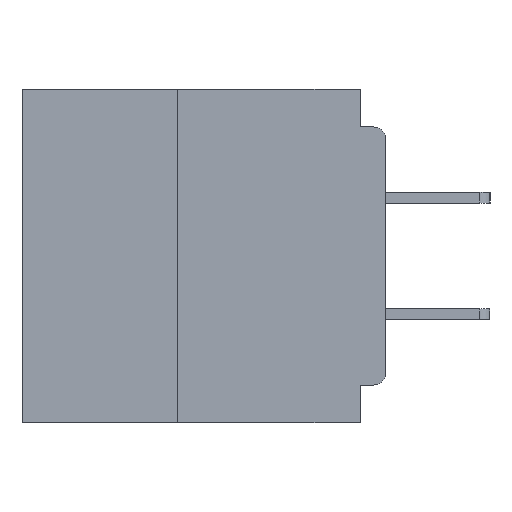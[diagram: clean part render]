
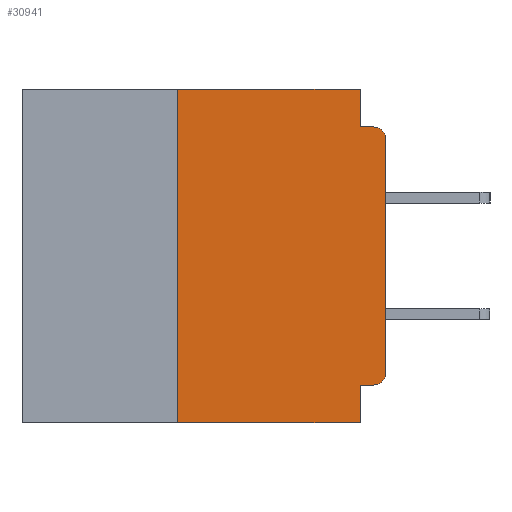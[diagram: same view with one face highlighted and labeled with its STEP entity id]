
A CAD part, left-side view. The second image highlights one B-rep face of the part: STEP entity #30941.
In plain terms, the highlighted planar face has unit normal (-1, 0, 0).
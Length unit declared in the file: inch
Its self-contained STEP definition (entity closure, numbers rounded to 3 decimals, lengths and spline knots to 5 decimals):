
#73 = EDGE_CURVE ( 'NONE', #10631, #47198, #45002, .T. ) ;
#103 = VERTEX_POINT ( 'NONE', #47614 ) ;
#166 = EDGE_CURVE ( 'NONE', #38303, #42740, #32128, .T. ) ;
#381 = ORIENTED_EDGE ( 'NONE', *, *, #36331, .F. ) ;
#466 = DIRECTION ( 'NONE',  ( 0., -1., 0. ) ) ;
#720 = EDGE_CURVE ( 'NONE', #40100, #45804, #36971, .T. ) ;
#778 = VECTOR ( 'NONE', #30493, 39.37008 ) ;
#966 = DIRECTION ( 'NONE',  ( 0., -1., 0. ) ) ;
#1097 = VERTEX_POINT ( 'NONE', #38771 ) ;
#1276 = LINE ( 'NONE', #42677, #31712 ) ;
#1330 = DIRECTION ( 'NONE',  ( -1., 0., 0. ) ) ;
#1372 = VERTEX_POINT ( 'NONE', #24798 ) ;
#2647 = DIRECTION ( 'NONE',  ( 0., 0., -1. ) ) ;
#2910 = ORIENTED_EDGE ( 'NONE', *, *, #73, .F. ) ;
#3764 = ORIENTED_EDGE ( 'NONE', *, *, #27282, .F. ) ;
#5622 = DIRECTION ( 'NONE',  ( 0., 0., 1. ) ) ;
#5649 = PLANE ( 'NONE',  #48093 ) ;
#5783 = CARTESIAN_POINT ( 'NONE',  ( 0., 0.25, -0.4 ) ) ;
#6669 = ORIENTED_EDGE ( 'NONE', *, *, #6833, .F. ) ;
#6833 = EDGE_CURVE ( 'NONE', #40100, #103, #1276, .T. ) ;
#9075 = VERTEX_POINT ( 'NONE', #46706 ) ;
#9662 = DIRECTION ( 'NONE',  ( 1., 0., 0. ) ) ;
#9680 = CARTESIAN_POINT ( 'NONE',  ( 0., 0., 0. ) ) ;
#10631 = VERTEX_POINT ( 'NONE', #31470 ) ;
#12347 = CARTESIAN_POINT ( 'NONE',  ( 0., 0.437, 0. ) ) ;
#13268 = CARTESIAN_POINT ( 'NONE',  ( 0., 0.437, -0.4 ) ) ;
#19511 = ORIENTED_EDGE ( 'NONE', *, *, #36813, .F. ) ;
#20322 = CARTESIAN_POINT ( 'NONE',  ( 0., 0.031, -0.4 ) ) ;
#23499 = LINE ( 'NONE', #5783, #43173 ) ;
#24798 = CARTESIAN_POINT ( 'NONE',  ( 0., 0.25, 0. ) ) ;
#24880 = ORIENTED_EDGE ( 'NONE', *, *, #720, .T. ) ;
#25169 = CARTESIAN_POINT ( 'NONE',  ( 0., 0.015, -0.06 ) ) ;
#25538 = DIRECTION ( 'NONE',  ( -1., 0., 0. ) ) ;
#26709 = VECTOR ( 'NONE', #37315, 39.37008 ) ;
#26934 = ORIENTED_EDGE ( 'NONE', *, *, #40611, .T. ) ;
#27282 = EDGE_CURVE ( 'NONE', #9075, #10631, #41637, .T. ) ;
#28320 = LINE ( 'NONE', #20322, #48008 ) ;
#28682 = AXIS2_PLACEMENT_3D ( 'NONE', #25169, #1330, #29096 ) ;
#28920 = EDGE_CURVE ( 'NONE', #45804, #1097, #38390, .T. ) ;
#29096 = DIRECTION ( 'NONE',  ( 0., 0., -1. ) ) ;
#29609 = VECTOR ( 'NONE', #466, 39.37008 ) ;
#29658 = CARTESIAN_POINT ( 'NONE',  ( 0., 0.015, -0.355 ) ) ;
#30235 = CARTESIAN_POINT ( 'NONE',  ( 0., 0.015, -0.045 ) ) ;
#30493 = DIRECTION ( 'NONE',  ( 0., 0., -1. ) ) ;
#30941 = ADVANCED_FACE ( 'NONE', ( #43107 ), #5649, .F. ) ;
#31470 = CARTESIAN_POINT ( 'NONE',  ( 0., 0.031, -0.045 ) ) ;
#31631 = EDGE_LOOP ( 'NONE', ( #38741, #26934, #2910, #3764, #381, #41489, #33627, #19511, #6669, #24880 ) ) ;
#31712 = VECTOR ( 'NONE', #38874, 39.37008 ) ;
#32128 = LINE ( 'NONE', #13268, #40053 ) ;
#33411 = CARTESIAN_POINT ( 'NONE',  ( 0., 0.437, 0. ) ) ;
#33627 = ORIENTED_EDGE ( 'NONE', *, *, #166, .T. ) ;
#34549 = VECTOR ( 'NONE', #47604, 39.37008 ) ;
#36331 = EDGE_CURVE ( 'NONE', #1372, #9075, #40046, .T. ) ;
#36813 = EDGE_CURVE ( 'NONE', #103, #42740, #28320, .T. ) ;
#36971 = CIRCLE ( 'NONE', #42866, 0.015 ) ;
#37301 = DIRECTION ( 'NONE',  ( 0., 0., -1. ) ) ;
#37315 = DIRECTION ( 'NONE',  ( 0., 0., 1. ) ) ;
#37717 = CARTESIAN_POINT ( 'NONE',  ( 0., 0.031, -0.4 ) ) ;
#38303 = VERTEX_POINT ( 'NONE', #48711 ) ;
#38319 = CARTESIAN_POINT ( 'NONE',  ( 0., 0.015, -0.34 ) ) ;
#38390 = LINE ( 'NONE', #9680, #26709 ) ;
#38741 = ORIENTED_EDGE ( 'NONE', *, *, #28920, .T. ) ;
#38771 = CARTESIAN_POINT ( 'NONE',  ( 0., 0., -0.06 ) ) ;
#38874 = DIRECTION ( 'NONE',  ( 0., 1., 0. ) ) ;
#39919 = DIRECTION ( 'NONE',  ( 0., 0., -1. ) ) ;
#40046 = LINE ( 'NONE', #12347, #29609 ) ;
#40053 = VECTOR ( 'NONE', #966, 39.37008 ) ;
#40100 = VERTEX_POINT ( 'NONE', #29658 ) ;
#40432 = CIRCLE ( 'NONE', #28682, 0.015 ) ;
#40611 = EDGE_CURVE ( 'NONE', #1097, #47198, #40432, .T. ) ;
#40981 = CARTESIAN_POINT ( 'NONE',  ( 0., 0., -0.34 ) ) ;
#41489 = ORIENTED_EDGE ( 'NONE', *, *, #43863, .F. ) ;
#41637 = LINE ( 'NONE', #42325, #778 ) ;
#42325 = CARTESIAN_POINT ( 'NONE',  ( 0., 0.031, 0. ) ) ;
#42677 = CARTESIAN_POINT ( 'NONE',  ( 0., 0., -0.355 ) ) ;
#42740 = VERTEX_POINT ( 'NONE', #37717 ) ;
#42866 = AXIS2_PLACEMENT_3D ( 'NONE', #38319, #25538, #2647 ) ;
#43107 = FACE_OUTER_BOUND ( 'NONE', #31631, .T. ) ;
#43173 = VECTOR ( 'NONE', #5622, 39.37008 ) ;
#43863 = EDGE_CURVE ( 'NONE', #38303, #1372, #23499, .T. ) ;
#45002 = LINE ( 'NONE', #51192, #34549 ) ;
#45804 = VERTEX_POINT ( 'NONE', #40981 ) ;
#46706 = CARTESIAN_POINT ( 'NONE',  ( 0., 0.031, 0. ) ) ;
#47198 = VERTEX_POINT ( 'NONE', #30235 ) ;
#47604 = DIRECTION ( 'NONE',  ( 0., -1., 0. ) ) ;
#47614 = CARTESIAN_POINT ( 'NONE',  ( 0., 0.031, -0.355 ) ) ;
#48008 = VECTOR ( 'NONE', #39919, 39.37008 ) ;
#48093 = AXIS2_PLACEMENT_3D ( 'NONE', #33411, #9662, #37301 ) ;
#48711 = CARTESIAN_POINT ( 'NONE',  ( 0., 0.25, -0.4 ) ) ;
#51192 = CARTESIAN_POINT ( 'NONE',  ( 0., 0., -0.045 ) ) ;
